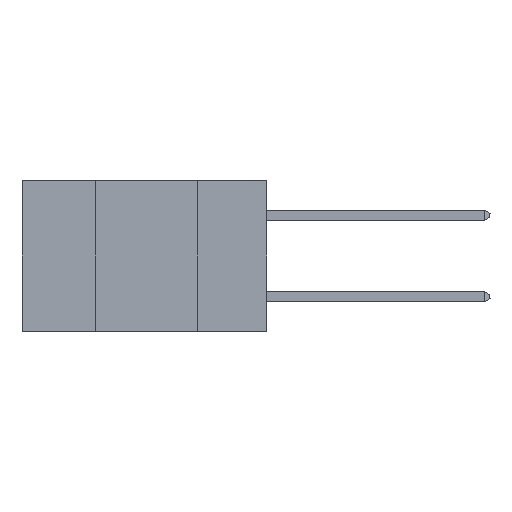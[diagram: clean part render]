
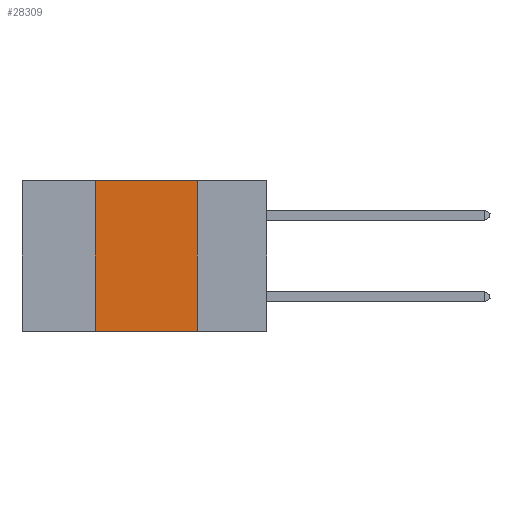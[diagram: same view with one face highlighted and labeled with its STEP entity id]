
A CAD part, left-side view. The second image highlights one B-rep face of the part: STEP entity #28309.
In plain terms, the highlighted planar face has unit normal (-1, 0, 0).
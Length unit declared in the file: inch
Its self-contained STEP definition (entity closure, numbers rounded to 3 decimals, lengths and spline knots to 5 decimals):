
#745 = CARTESIAN_POINT ( 'NONE',  ( 0., 0.17, 0. ) ) ;
#2185 = LINE ( 'NONE', #35555, #44082 ) ;
#3853 = LINE ( 'NONE', #9945, #52038 ) ;
#4488 = DIRECTION ( 'NONE',  ( 0., 0., -1. ) ) ;
#6665 = CARTESIAN_POINT ( 'NONE',  ( 0., 0.6, 0. ) ) ;
#8097 = CARTESIAN_POINT ( 'NONE',  ( 0., 0.42, 0. ) ) ;
#8177 = CARTESIAN_POINT ( 'NONE',  ( 0., 0.17, 0. ) ) ;
#9945 = CARTESIAN_POINT ( 'NONE',  ( 0., 0.6, -0.37 ) ) ;
#10991 = EDGE_LOOP ( 'NONE', ( #14559, #42919, #18998, #35358 ) ) ;
#14373 = DIRECTION ( 'NONE',  ( 0., -1., 0. ) ) ;
#14559 = ORIENTED_EDGE ( 'NONE', *, *, #31128, .F. ) ;
#14793 = EDGE_CURVE ( 'NONE', #47418, #18523, #15291, .T. ) ;
#15291 = LINE ( 'NONE', #37040, #35584 ) ;
#18523 = VERTEX_POINT ( 'NONE', #8097 ) ;
#18998 = ORIENTED_EDGE ( 'NONE', *, *, #14793, .F. ) ;
#19056 = EDGE_CURVE ( 'NONE', #18523, #48144, #2185, .T. ) ;
#27061 = DIRECTION ( 'NONE',  ( 1., 0., 0. ) ) ;
#27090 = EDGE_CURVE ( 'NONE', #47418, #47692, #3853, .T. ) ;
#28309 = ADVANCED_FACE ( 'NONE', ( #32321 ), #39434, .F. ) ;
#31128 = EDGE_CURVE ( 'NONE', #48144, #47692, #40031, .T. ) ;
#32321 = FACE_OUTER_BOUND ( 'NONE', #10991, .T. ) ;
#33971 = CARTESIAN_POINT ( 'NONE',  ( 0., 0.17, -0.37 ) ) ;
#35358 = ORIENTED_EDGE ( 'NONE', *, *, #27090, .T. ) ;
#35555 = CARTESIAN_POINT ( 'NONE',  ( 0., 0.6, 0. ) ) ;
#35584 = VECTOR ( 'NONE', #37220, 39.37008 ) ;
#37040 = CARTESIAN_POINT ( 'NONE',  ( 0., 0.42, 0. ) ) ;
#37220 = DIRECTION ( 'NONE',  ( 0., 0., 1. ) ) ;
#39242 = DIRECTION ( 'NONE',  ( 0., -1., 0. ) ) ;
#39434 = PLANE ( 'NONE',  #52020 ) ;
#40031 = LINE ( 'NONE', #745, #43190 ) ;
#42919 = ORIENTED_EDGE ( 'NONE', *, *, #19056, .F. ) ;
#43190 = VECTOR ( 'NONE', #4488, 39.37008 ) ;
#44082 = VECTOR ( 'NONE', #39242, 39.37008 ) ;
#47401 = DIRECTION ( 'NONE',  ( 0., 0., -1. ) ) ;
#47418 = VERTEX_POINT ( 'NONE', #47836 ) ;
#47692 = VERTEX_POINT ( 'NONE', #33971 ) ;
#47836 = CARTESIAN_POINT ( 'NONE',  ( 0., 0.42, -0.37 ) ) ;
#48144 = VERTEX_POINT ( 'NONE', #8177 ) ;
#52020 = AXIS2_PLACEMENT_3D ( 'NONE', #6665, #27061, #47401 ) ;
#52038 = VECTOR ( 'NONE', #14373, 39.37008 ) ;
